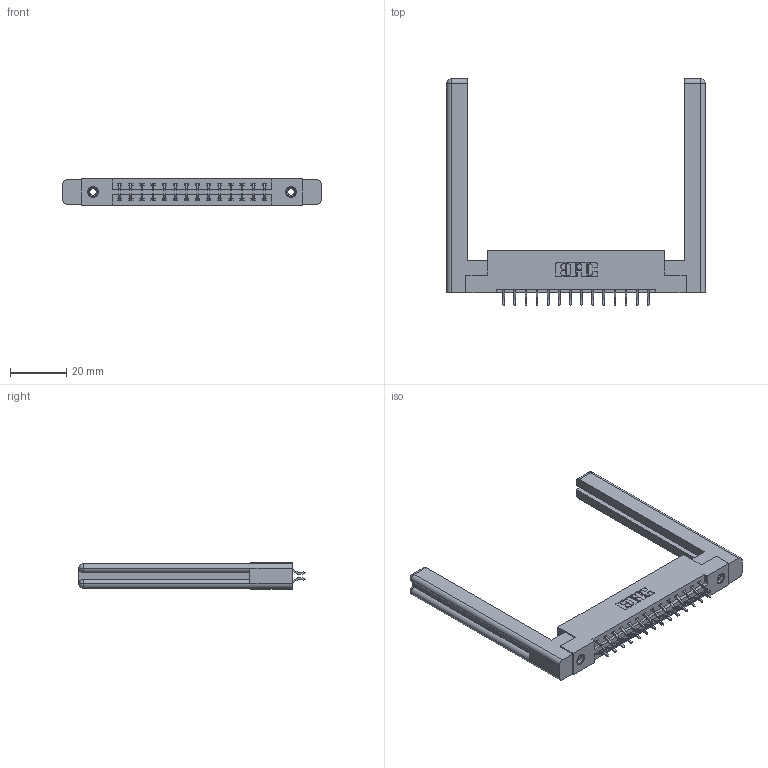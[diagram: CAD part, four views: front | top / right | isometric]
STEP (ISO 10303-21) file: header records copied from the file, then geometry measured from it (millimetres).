
FILE_DESCRIPTION (( 'STEP AP203' ), '1' );
FILE_NAME ('387-028-556-258.STEP', '2019-10-16T22:49:33', ( '' ), ( '' ), 'SwSTEP 2.0', 'SolidWorks 2016', '' );
FILE_SCHEMA (( 'CONFIG_CONTROL_DESIGN' ));
Length unit declared in the file: inch
Products named in the file (5): 345-292-001_556 Tail; 387-028-556-258; 337 Part_Flush Mounting Lugs - 0.156 Dia-TI; 345-250-001_345-250-001-102; 307-220-058
Assembly tree (33 placements, depth 2):
  387-028-556-258
    337 Part_Flush Mounting Lugs - 0.156 Dia-TI
    345-292-001_556 Tail  x28
    345-250-001_345-250-001-102  x2
    307-220-058  x2
Bounding box: 92.1 x 80.66 x 9.4 mm (x, y, z)
Volume: 16474.8 mm3; surface area: 15295.6 mm2
Topology: 33 solids, 33 shells, 1936 faces, 5677 edges, 3734 vertices
Faces by surface type: plane 1330, cylinder 582, cone 12, torus 12
Entity records: 17330 total; most frequent: CARTESIAN_POINT 2965, ORIENTED_EDGE 2828, DIRECTION 2578, EDGE_CURVE 1414, LINE 1230, VECTOR 1230, VERTEX_POINT 934, AXIS2_PLACEMENT_3D 674
